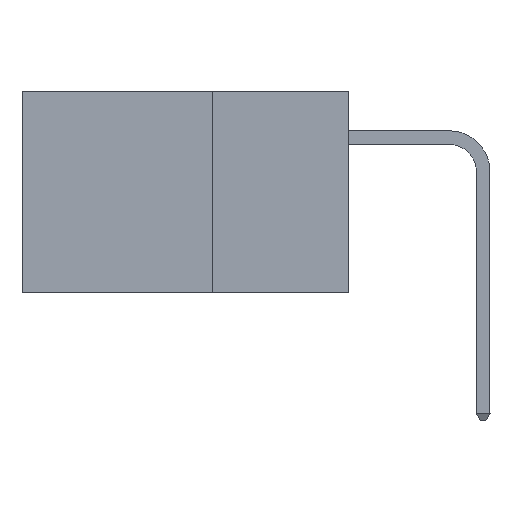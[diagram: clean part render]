
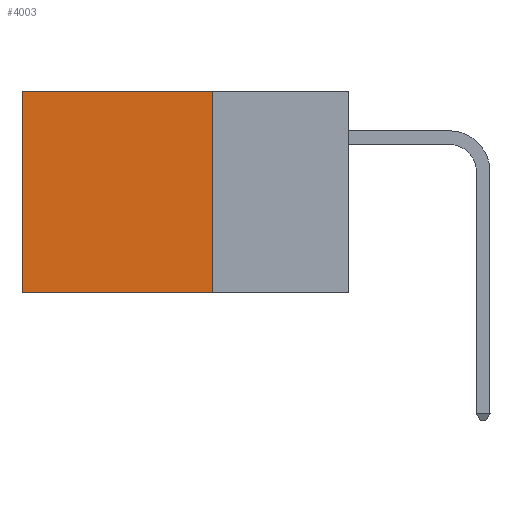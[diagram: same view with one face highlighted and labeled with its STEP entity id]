
A CAD part, left-side view. The second image highlights one B-rep face of the part: STEP entity #4003.
In plain terms, the highlighted planar face has unit normal (-1, 0, 0).
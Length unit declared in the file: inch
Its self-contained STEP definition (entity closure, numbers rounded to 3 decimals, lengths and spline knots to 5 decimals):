
#61 = DIRECTION ( 'NONE',  ( 0., 0., -1. ) ) ;
#914 = LINE ( 'NONE', #15515, #22810 ) ;
#1586 = PLANE ( 'NONE',  #14675 ) ;
#3196 = VERTEX_POINT ( 'NONE', #5221 ) ;
#4003 = ADVANCED_FACE ( 'NONE', ( #10724 ), #1586, .F. ) ;
#5116 = VECTOR ( 'NONE', #21187, 39.37008 ) ;
#5138 = CARTESIAN_POINT ( 'NONE',  ( 0.2875, 0.25, 0. ) ) ;
#5221 = CARTESIAN_POINT ( 'NONE',  ( 0.2875, 0.25, -0.37 ) ) ;
#5524 = DIRECTION ( 'NONE',  ( 0., 1., 0. ) ) ;
#7650 = EDGE_CURVE ( 'NONE', #7953, #10189, #20116, .T. ) ;
#7953 = VERTEX_POINT ( 'NONE', #15820 ) ;
#8268 = CARTESIAN_POINT ( 'NONE',  ( 0.2875, 0.25, 0. ) ) ;
#8844 = LINE ( 'NONE', #18106, #12672 ) ;
#10189 = VERTEX_POINT ( 'NONE', #12646 ) ;
#10617 = VECTOR ( 'NONE', #61, 39.37008 ) ;
#10724 = FACE_OUTER_BOUND ( 'NONE', #18710, .T. ) ;
#10960 = VERTEX_POINT ( 'NONE', #8268 ) ;
#11063 = ORIENTED_EDGE ( 'NONE', *, *, #19242, .F. ) ;
#12646 = CARTESIAN_POINT ( 'NONE',  ( 0.2875, 0.6, -0.37 ) ) ;
#12672 = VECTOR ( 'NONE', #5524, 39.37008 ) ;
#13070 = ORIENTED_EDGE ( 'NONE', *, *, #16360, .F. ) ;
#14011 = EDGE_CURVE ( 'NONE', #10960, #7953, #914, .T. ) ;
#14675 = AXIS2_PLACEMENT_3D ( 'NONE', #5138, #19754, #15954 ) ;
#15515 = CARTESIAN_POINT ( 'NONE',  ( 0.2875, 0.25, 0. ) ) ;
#15820 = CARTESIAN_POINT ( 'NONE',  ( 0.2875, 0.6, 0. ) ) ;
#15954 = DIRECTION ( 'NONE',  ( 0., 0., -1. ) ) ;
#15965 = CARTESIAN_POINT ( 'NONE',  ( 0.2875, 0.6, 0. ) ) ;
#16360 = EDGE_CURVE ( 'NONE', #3196, #10189, #8844, .T. ) ;
#18106 = CARTESIAN_POINT ( 'NONE',  ( 0.2875, 0.25, -0.37 ) ) ;
#18710 = EDGE_LOOP ( 'NONE', ( #22868, #13070, #11063, #22451 ) ) ;
#19242 = EDGE_CURVE ( 'NONE', #10960, #3196, #23083, .T. ) ;
#19754 = DIRECTION ( 'NONE',  ( 1., 0., 0. ) ) ;
#20116 = LINE ( 'NONE', #15965, #10617 ) ;
#21101 = DIRECTION ( 'NONE',  ( 0., 1., 0. ) ) ;
#21187 = DIRECTION ( 'NONE',  ( 0., 0., -1. ) ) ;
#22451 = ORIENTED_EDGE ( 'NONE', *, *, #14011, .T. ) ;
#22810 = VECTOR ( 'NONE', #21101, 39.37008 ) ;
#22868 = ORIENTED_EDGE ( 'NONE', *, *, #7650, .T. ) ;
#23083 = LINE ( 'NONE', #23201, #5116 ) ;
#23201 = CARTESIAN_POINT ( 'NONE',  ( 0.2875, 0.25, 0. ) ) ;
